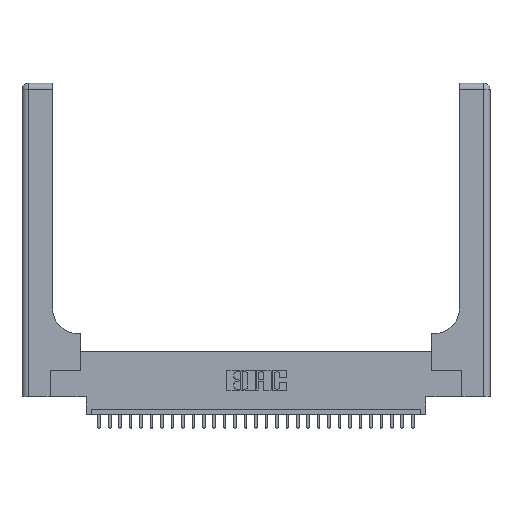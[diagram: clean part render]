
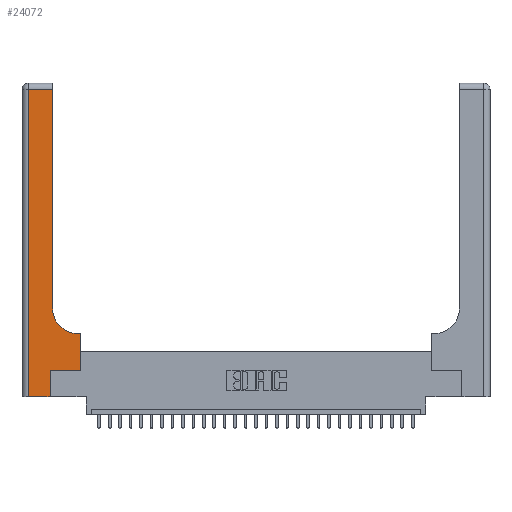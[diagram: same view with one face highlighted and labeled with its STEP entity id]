
A CAD part, top view. The second image highlights one B-rep face of the part: STEP entity #24072.
In plain terms, the highlighted planar face has unit normal (0, 0, 1).
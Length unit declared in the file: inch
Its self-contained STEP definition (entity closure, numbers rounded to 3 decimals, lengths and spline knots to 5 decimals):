
#146 = CARTESIAN_POINT ( 'NONE',  ( 0.5415, 0.6, 0.37 ) ) ;
#384 = CARTESIAN_POINT ( 'NONE',  ( 0., 2.94, 0.37 ) ) ;
#431 = CARTESIAN_POINT ( 'NONE',  ( 0.5585, 0.6, 0.37 ) ) ;
#876 = CARTESIAN_POINT ( 'NONE',  ( 0.269, 0., 0.37 ) ) ;
#883 = LINE ( 'NONE', #384, #12501 ) ;
#1073 = VECTOR ( 'NONE', #22044, 39.37008 ) ;
#1287 = ORIENTED_EDGE ( 'NONE', *, *, #6214, .T. ) ;
#1388 = CARTESIAN_POINT ( 'NONE',  ( 0.2915, 0.85, 0.37 ) ) ;
#1442 = LINE ( 'NONE', #5065, #19971 ) ;
#1513 = VERTEX_POINT ( 'NONE', #1388 ) ;
#2242 = VECTOR ( 'NONE', #5774, 39.37008 ) ;
#2562 = EDGE_CURVE ( 'NONE', #24150, #26591, #5718, .T. ) ;
#3217 = CARTESIAN_POINT ( 'NONE',  ( 0.5585, 0.25, 0.37 ) ) ;
#3319 = VECTOR ( 'NONE', #24475, 39.37008 ) ;
#3380 = CARTESIAN_POINT ( 'NONE',  ( 0.269, 0., 0.37 ) ) ;
#3702 = LINE ( 'NONE', #3217, #2242 ) ;
#4571 = EDGE_CURVE ( 'NONE', #22797, #5763, #15800, .T. ) ;
#4884 = VECTOR ( 'NONE', #26201, 39.37008 ) ;
#5065 = CARTESIAN_POINT ( 'NONE',  ( 0.2915, 3., 0.37 ) ) ;
#5123 = CARTESIAN_POINT ( 'NONE',  ( 0., 0., 0.37 ) ) ;
#5161 = DIRECTION ( 'NONE',  ( -1., 0., 0. ) ) ;
#5647 = EDGE_LOOP ( 'NONE', ( #8706, #13652, #26208, #11733, #15886, #28750, #7147, #26782, #1287 ) ) ;
#5718 = LINE ( 'NONE', #19920, #11158 ) ;
#5758 = PLANE ( 'NONE',  #13483 ) ;
#5763 = VERTEX_POINT ( 'NONE', #26187 ) ;
#5774 = DIRECTION ( 'NONE',  ( 0., 1., 0. ) ) ;
#6206 = EDGE_CURVE ( 'NONE', #10149, #6970, #16393, .T. ) ;
#6214 = EDGE_CURVE ( 'NONE', #26591, #1513, #14202, .T. ) ;
#6970 = VERTEX_POINT ( 'NONE', #29865 ) ;
#7079 = FACE_OUTER_BOUND ( 'NONE', #5647, .T. ) ;
#7147 = ORIENTED_EDGE ( 'NONE', *, *, #19976, .T. ) ;
#7275 = CARTESIAN_POINT ( 'NONE',  ( 0.2915, 2.94, 0.37 ) ) ;
#7324 = VERTEX_POINT ( 'NONE', #17477 ) ;
#8706 = ORIENTED_EDGE ( 'NONE', *, *, #9937, .T. ) ;
#9937 = EDGE_CURVE ( 'NONE', #1513, #27271, #1442, .T. ) ;
#10149 = VERTEX_POINT ( 'NONE', #20173 ) ;
#10419 = DIRECTION ( 'NONE',  ( -1., 0., 0. ) ) ;
#11158 = VECTOR ( 'NONE', #26672, 39.37008 ) ;
#11188 = DIRECTION ( 'NONE',  ( 1., 0., 0. ) ) ;
#11733 = ORIENTED_EDGE ( 'NONE', *, *, #21117, .T. ) ;
#12501 = VECTOR ( 'NONE', #5161, 39.37008 ) ;
#12877 = VECTOR ( 'NONE', #24995, 39.37008 ) ;
#13483 = AXIS2_PLACEMENT_3D ( 'NONE', #21999, #24396, #10419 ) ;
#13652 = ORIENTED_EDGE ( 'NONE', *, *, #24977, .T. ) ;
#14202 = CIRCLE ( 'NONE', #24254, 0.25 ) ;
#15092 = CARTESIAN_POINT ( 'NONE',  ( 0.06, 3., 0.37 ) ) ;
#15473 = EDGE_CURVE ( 'NONE', #5763, #7324, #22864, .T. ) ;
#15800 = LINE ( 'NONE', #876, #12877 ) ;
#15886 = ORIENTED_EDGE ( 'NONE', *, *, #4571, .T. ) ;
#16393 = LINE ( 'NONE', #15092, #3319 ) ;
#17477 = CARTESIAN_POINT ( 'NONE',  ( 0.5585, 0.25, 0.37 ) ) ;
#19081 = DIRECTION ( 'NONE',  ( 0., 1., 0. ) ) ;
#19920 = CARTESIAN_POINT ( 'NONE',  ( 0.2915, 0.6, 0.37 ) ) ;
#19971 = VECTOR ( 'NONE', #19081, 39.37008 ) ;
#19974 = LINE ( 'NONE', #5123, #4884 ) ;
#19976 = EDGE_CURVE ( 'NONE', #7324, #24150, #3702, .T. ) ;
#20173 = CARTESIAN_POINT ( 'NONE',  ( 0.06, 2.94, 0.37 ) ) ;
#21117 = EDGE_CURVE ( 'NONE', #6970, #22797, #19974, .T. ) ;
#21999 = CARTESIAN_POINT ( 'NONE',  ( 0., 3., 0.37 ) ) ;
#22044 = DIRECTION ( 'NONE',  ( 1., 0., 0. ) ) ;
#22401 = CARTESIAN_POINT ( 'NONE',  ( 0.5415, 0.85, 0.37 ) ) ;
#22510 = DIRECTION ( 'NONE',  ( 0., 0., -1. ) ) ;
#22797 = VERTEX_POINT ( 'NONE', #3380 ) ;
#22864 = LINE ( 'NONE', #26046, #1073 ) ;
#24072 = ADVANCED_FACE ( 'NONE', ( #7079 ), #5758, .F. ) ;
#24150 = VERTEX_POINT ( 'NONE', #431 ) ;
#24254 = AXIS2_PLACEMENT_3D ( 'NONE', #22401, #22510, #11188 ) ;
#24396 = DIRECTION ( 'NONE',  ( 0., 0., -1. ) ) ;
#24475 = DIRECTION ( 'NONE',  ( 0., -1., 0. ) ) ;
#24977 = EDGE_CURVE ( 'NONE', #27271, #10149, #883, .T. ) ;
#24995 = DIRECTION ( 'NONE',  ( 0., 1., 0. ) ) ;
#26046 = CARTESIAN_POINT ( 'NONE',  ( 0.269, 0.25, 0.37 ) ) ;
#26187 = CARTESIAN_POINT ( 'NONE',  ( 0.269, 0.25, 0.37 ) ) ;
#26201 = DIRECTION ( 'NONE',  ( 1., 0., 0. ) ) ;
#26208 = ORIENTED_EDGE ( 'NONE', *, *, #6206, .T. ) ;
#26591 = VERTEX_POINT ( 'NONE', #146 ) ;
#26672 = DIRECTION ( 'NONE',  ( -1., 0., 0. ) ) ;
#26782 = ORIENTED_EDGE ( 'NONE', *, *, #2562, .T. ) ;
#27271 = VERTEX_POINT ( 'NONE', #7275 ) ;
#28750 = ORIENTED_EDGE ( 'NONE', *, *, #15473, .T. ) ;
#29865 = CARTESIAN_POINT ( 'NONE',  ( 0.06, 0., 0.37 ) ) ;
